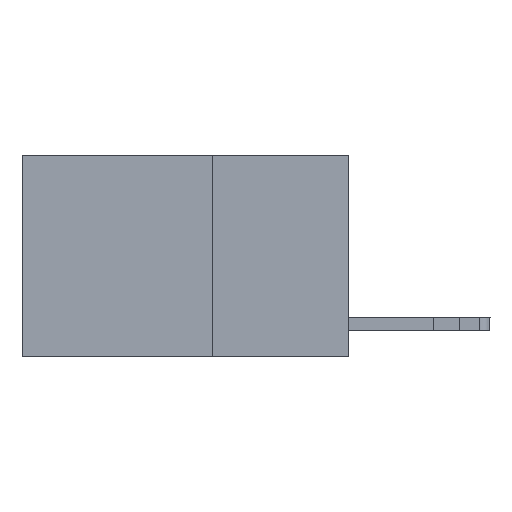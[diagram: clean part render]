
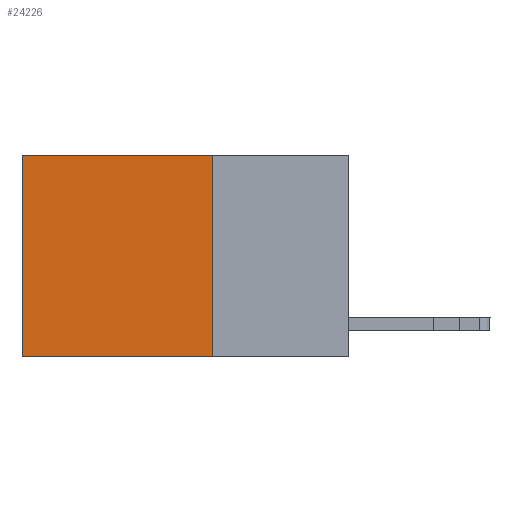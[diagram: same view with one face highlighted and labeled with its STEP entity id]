
A CAD part, left-side view. The second image highlights one B-rep face of the part: STEP entity #24226.
In plain terms, the highlighted planar face has unit normal (-1, 0, 0).
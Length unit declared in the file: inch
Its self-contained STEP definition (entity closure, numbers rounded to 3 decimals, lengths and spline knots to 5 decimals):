
#878 = CARTESIAN_POINT ( 'NONE',  ( 0.2625, 0.25, 0. ) ) ;
#2045 = EDGE_CURVE ( 'NONE', #10331, #12583, #16756, .T. ) ;
#2484 = CARTESIAN_POINT ( 'NONE',  ( 0.2625, 0.25, 0. ) ) ;
#2982 = ORIENTED_EDGE ( 'NONE', *, *, #17838, .F. ) ;
#3893 = EDGE_LOOP ( 'NONE', ( #13192, #5839, #2982, #20564 ) ) ;
#4118 = LINE ( 'NONE', #878, #23538 ) ;
#5115 = CARTESIAN_POINT ( 'NONE',  ( 0.2625, 0.6, 0. ) ) ;
#5739 = CARTESIAN_POINT ( 'NONE',  ( 0.2625, 0.25, -0.37 ) ) ;
#5839 = ORIENTED_EDGE ( 'NONE', *, *, #24212, .F. ) ;
#6872 = DIRECTION ( 'NONE',  ( 0., 1., 0. ) ) ;
#8836 = PLANE ( 'NONE',  #15279 ) ;
#8968 = VERTEX_POINT ( 'NONE', #5739 ) ;
#9204 = LINE ( 'NONE', #18371, #13744 ) ;
#10331 = VERTEX_POINT ( 'NONE', #5115 ) ;
#10631 = CARTESIAN_POINT ( 'NONE',  ( 0.2625, 0.25, 0. ) ) ;
#10803 = DIRECTION ( 'NONE',  ( 1., 0., 0. ) ) ;
#11167 = DIRECTION ( 'NONE',  ( 0., 0., -1. ) ) ;
#12583 = VERTEX_POINT ( 'NONE', #15964 ) ;
#13192 = ORIENTED_EDGE ( 'NONE', *, *, #2045, .T. ) ;
#13744 = VECTOR ( 'NONE', #20267, 39.37008 ) ;
#14299 = VECTOR ( 'NONE', #16184, 39.37008 ) ;
#15279 = AXIS2_PLACEMENT_3D ( 'NONE', #10631, #10803, #24235 ) ;
#15964 = CARTESIAN_POINT ( 'NONE',  ( 0.2625, 0.6, -0.37 ) ) ;
#16184 = DIRECTION ( 'NONE',  ( 0., 0., -1. ) ) ;
#16756 = LINE ( 'NONE', #16901, #21242 ) ;
#16901 = CARTESIAN_POINT ( 'NONE',  ( 0.2625, 0.6, 0. ) ) ;
#17838 = EDGE_CURVE ( 'NONE', #24590, #8968, #23905, .T. ) ;
#18258 = FACE_OUTER_BOUND ( 'NONE', #3893, .T. ) ;
#18371 = CARTESIAN_POINT ( 'NONE',  ( 0.2625, 0.25, -0.37 ) ) ;
#18870 = EDGE_CURVE ( 'NONE', #24590, #10331, #4118, .T. ) ;
#20267 = DIRECTION ( 'NONE',  ( 0., 1., 0. ) ) ;
#20564 = ORIENTED_EDGE ( 'NONE', *, *, #18870, .T. ) ;
#21242 = VECTOR ( 'NONE', #11167, 39.37008 ) ;
#21467 = CARTESIAN_POINT ( 'NONE',  ( 0.2625, 0.25, 0. ) ) ;
#23538 = VECTOR ( 'NONE', #6872, 39.37008 ) ;
#23905 = LINE ( 'NONE', #2484, #14299 ) ;
#24212 = EDGE_CURVE ( 'NONE', #8968, #12583, #9204, .T. ) ;
#24226 = ADVANCED_FACE ( 'NONE', ( #18258 ), #8836, .F. ) ;
#24235 = DIRECTION ( 'NONE',  ( 0., 0., -1. ) ) ;
#24590 = VERTEX_POINT ( 'NONE', #21467 ) ;
